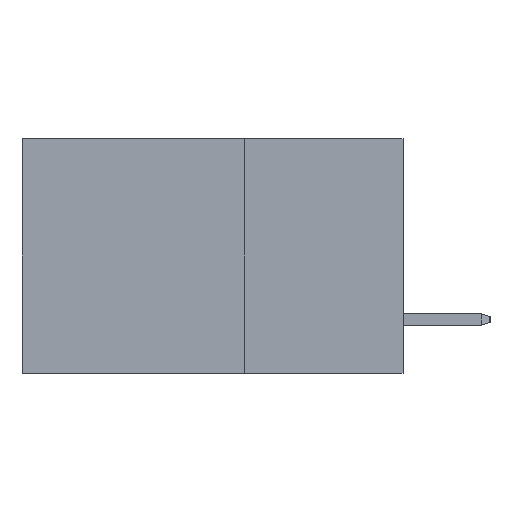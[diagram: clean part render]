
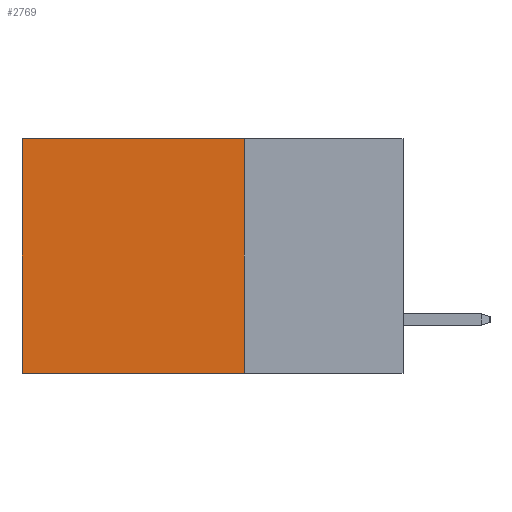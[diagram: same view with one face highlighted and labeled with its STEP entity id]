
A CAD part, left-side view. The second image highlights one B-rep face of the part: STEP entity #2769.
In plain terms, the highlighted planar face has unit normal (-1, 0, 0).
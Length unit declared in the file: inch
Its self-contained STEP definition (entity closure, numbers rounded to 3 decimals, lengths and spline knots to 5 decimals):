
#60 = CARTESIAN_POINT ( 'NONE',  ( 0.2875, 0.25, 0. ) ) ;
#80 = DIRECTION ( 'NONE',  ( 0., 1., 0. ) ) ;
#222 = LINE ( 'NONE', #10194, #1192 ) ;
#1192 = VECTOR ( 'NONE', #80, 39.37008 ) ;
#1252 = VERTEX_POINT ( 'NONE', #9025 ) ;
#1297 = CARTESIAN_POINT ( 'NONE',  ( 0.2875, 0.25, 0. ) ) ;
#1487 = ORIENTED_EDGE ( 'NONE', *, *, #6504, .T. ) ;
#1924 = VECTOR ( 'NONE', #10316, 39.37008 ) ;
#2167 = PLANE ( 'NONE',  #3257 ) ;
#2288 = ORIENTED_EDGE ( 'NONE', *, *, #13701, .F. ) ;
#2769 = ADVANCED_FACE ( 'NONE', ( #3617 ), #2167, .F. ) ;
#2794 = DIRECTION ( 'NONE',  ( 1., 0., 0. ) ) ;
#3185 = LINE ( 'NONE', #10846, #4283 ) ;
#3257 = AXIS2_PLACEMENT_3D ( 'NONE', #1297, #2794, #6094 ) ;
#3617 = FACE_OUTER_BOUND ( 'NONE', #12911, .T. ) ;
#4283 = VECTOR ( 'NONE', #12087, 39.37008 ) ;
#4479 = CARTESIAN_POINT ( 'NONE',  ( 0.2875, 0.6, 0. ) ) ;
#4844 = LINE ( 'NONE', #7177, #1924 ) ;
#5436 = LINE ( 'NONE', #4479, #6079 ) ;
#6079 = VECTOR ( 'NONE', #9881, 39.37008 ) ;
#6094 = DIRECTION ( 'NONE',  ( 0., 0., -1. ) ) ;
#6504 = EDGE_CURVE ( 'NONE', #6985, #9382, #222, .T. ) ;
#6985 = VERTEX_POINT ( 'NONE', #60 ) ;
#7177 = CARTESIAN_POINT ( 'NONE',  ( 0.2875, 0.25, -0.37 ) ) ;
#8657 = CARTESIAN_POINT ( 'NONE',  ( 0.2875, 0.6, 0. ) ) ;
#8698 = EDGE_CURVE ( 'NONE', #9382, #13247, #5436, .T. ) ;
#9025 = CARTESIAN_POINT ( 'NONE',  ( 0.2875, 0.25, -0.37 ) ) ;
#9071 = ORIENTED_EDGE ( 'NONE', *, *, #8698, .T. ) ;
#9382 = VERTEX_POINT ( 'NONE', #8657 ) ;
#9881 = DIRECTION ( 'NONE',  ( 0., 0., -1. ) ) ;
#10040 = EDGE_CURVE ( 'NONE', #1252, #13247, #4844, .T. ) ;
#10194 = CARTESIAN_POINT ( 'NONE',  ( 0.2875, 0.25, 0. ) ) ;
#10316 = DIRECTION ( 'NONE',  ( 0., 1., 0. ) ) ;
#10846 = CARTESIAN_POINT ( 'NONE',  ( 0.2875, 0.25, 0. ) ) ;
#10954 = CARTESIAN_POINT ( 'NONE',  ( 0.2875, 0.6, -0.37 ) ) ;
#12087 = DIRECTION ( 'NONE',  ( 0., 0., -1. ) ) ;
#12911 = EDGE_LOOP ( 'NONE', ( #9071, #12983, #2288, #1487 ) ) ;
#12983 = ORIENTED_EDGE ( 'NONE', *, *, #10040, .F. ) ;
#13247 = VERTEX_POINT ( 'NONE', #10954 ) ;
#13701 = EDGE_CURVE ( 'NONE', #6985, #1252, #3185, .T. ) ;
